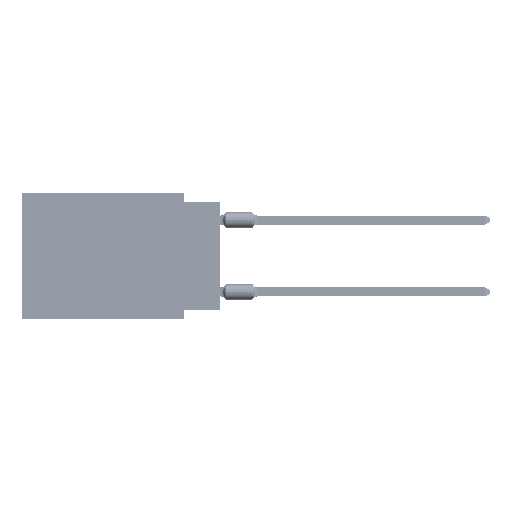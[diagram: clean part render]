
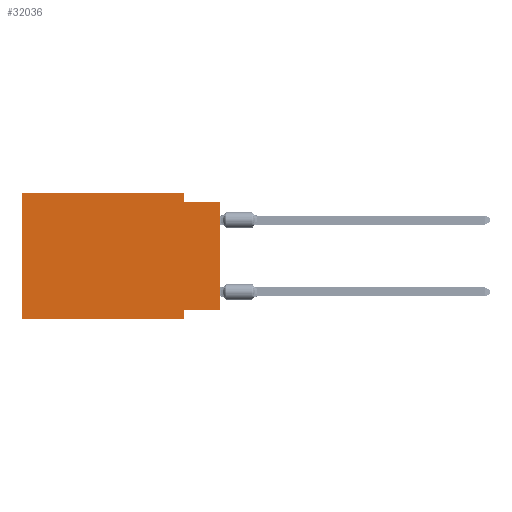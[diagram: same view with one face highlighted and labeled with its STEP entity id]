
A CAD part, left-side view. The second image highlights one B-rep face of the part: STEP entity #32036.
In plain terms, the highlighted planar face has unit normal (-1, 0, 0).
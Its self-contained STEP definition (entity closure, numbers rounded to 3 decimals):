
#431 = EDGE_CURVE ( 'NONE', #12247, #24004, #106293, .T. ) ;
#2744 = LINE ( 'NONE', #40920, #111306 ) ;
#5937 = DIRECTION ( 'NONE',  ( 0., -1., 0. ) ) ;
#11115 = CARTESIAN_POINT ( 'NONE',  ( 0., 0., -0.635 ) ) ;
#11215 = VERTEX_POINT ( 'NONE', #73390 ) ;
#11297 = VECTOR ( 'NONE', #75591, 1000. ) ;
#12247 = VERTEX_POINT ( 'NONE', #87187 ) ;
#15768 = CARTESIAN_POINT ( 'NONE',  ( 0., 13.97, 0. ) ) ;
#18069 = EDGE_CURVE ( 'NONE', #34538, #65398, #113765, .T. ) ;
#20602 = FACE_OUTER_BOUND ( 'NONE', #29272, .T. ) ;
#21909 = DIRECTION ( 'NONE',  ( 0., 0., 1. ) ) ;
#23655 = DIRECTION ( 'NONE',  ( 0., 0., -1. ) ) ;
#24004 = VERTEX_POINT ( 'NONE', #77155 ) ;
#27257 = ORIENTED_EDGE ( 'NONE', *, *, #98358, .F. ) ;
#28220 = LINE ( 'NONE', #68195, #44627 ) ;
#29272 = EDGE_LOOP ( 'NONE', ( #40018, #65477, #35209, #44432, #27257, #119231, #104005, #34527 ) ) ;
#30607 = CARTESIAN_POINT ( 'NONE',  ( 0., 13.97, 0. ) ) ;
#32036 = ADVANCED_FACE ( 'NONE', ( #20602 ), #96289, .F. ) ;
#32522 = CARTESIAN_POINT ( 'NONE',  ( 0., 0., -8.255 ) ) ;
#32680 = CARTESIAN_POINT ( 'NONE',  ( 0., 2.54, 0. ) ) ;
#34527 = ORIENTED_EDGE ( 'NONE', *, *, #18069, .F. ) ;
#34538 = VERTEX_POINT ( 'NONE', #32522 ) ;
#35209 = ORIENTED_EDGE ( 'NONE', *, *, #67756, .F. ) ;
#35765 = VECTOR ( 'NONE', #70231, 1000. ) ;
#39027 = VECTOR ( 'NONE', #5937, 1000. ) ;
#39082 = DIRECTION ( 'NONE',  ( 0., 0., -1. ) ) ;
#40018 = ORIENTED_EDGE ( 'NONE', *, *, #86306, .T. ) ;
#40446 = DIRECTION ( 'NONE',  ( 0., -1., 0. ) ) ;
#40472 = VERTEX_POINT ( 'NONE', #11115 ) ;
#40532 = CARTESIAN_POINT ( 'NONE',  ( 0., 2.54, -0.635 ) ) ;
#40920 = CARTESIAN_POINT ( 'NONE',  ( 0., 2.54, -8.89 ) ) ;
#43041 = VERTEX_POINT ( 'NONE', #73592 ) ;
#44149 = CARTESIAN_POINT ( 'NONE',  ( 0., 2.54, -8.255 ) ) ;
#44432 = ORIENTED_EDGE ( 'NONE', *, *, #431, .F. ) ;
#44627 = VECTOR ( 'NONE', #105753, 1000. ) ;
#47868 = VECTOR ( 'NONE', #40446, 1000. ) ;
#49040 = CARTESIAN_POINT ( 'NONE',  ( 0., 0., 0. ) ) ;
#50225 = LINE ( 'NONE', #49040, #109811 ) ;
#51982 = VERTEX_POINT ( 'NONE', #40532 ) ;
#54453 = AXIS2_PLACEMENT_3D ( 'NONE', #77192, #76007, #39082 ) ;
#60740 = EDGE_CURVE ( 'NONE', #65398, #43041, #2744, .T. ) ;
#61965 = LINE ( 'NONE', #99494, #39027 ) ;
#65398 = VERTEX_POINT ( 'NONE', #44149 ) ;
#65477 = ORIENTED_EDGE ( 'NONE', *, *, #99718, .F. ) ;
#67756 = EDGE_CURVE ( 'NONE', #24004, #51982, #88086, .T. ) ;
#68195 = CARTESIAN_POINT ( 'NONE',  ( 0., 13.97, -8.89 ) ) ;
#70231 = DIRECTION ( 'NONE',  ( 0., 0., -1. ) ) ;
#70576 = DIRECTION ( 'NONE',  ( 0., 0., 1. ) ) ;
#73390 = CARTESIAN_POINT ( 'NONE',  ( 0., 13.97, -8.89 ) ) ;
#73592 = CARTESIAN_POINT ( 'NONE',  ( 0., 2.54, -8.89 ) ) ;
#75591 = DIRECTION ( 'NONE',  ( 0., 1., 0. ) ) ;
#76007 = DIRECTION ( 'NONE',  ( 1., 0., 0. ) ) ;
#77155 = CARTESIAN_POINT ( 'NONE',  ( 0., 2.54, 0. ) ) ;
#77192 = CARTESIAN_POINT ( 'NONE',  ( 0., 13.97, 0. ) ) ;
#82605 = EDGE_CURVE ( 'NONE', #11215, #43041, #28220, .T. ) ;
#86306 = EDGE_CURVE ( 'NONE', #34538, #40472, #50225, .T. ) ;
#87187 = CARTESIAN_POINT ( 'NONE',  ( 0., 13.97, 0. ) ) ;
#88086 = LINE ( 'NONE', #32680, #35765 ) ;
#96289 = PLANE ( 'NONE',  #54453 ) ;
#98358 = EDGE_CURVE ( 'NONE', #11215, #12247, #100084, .T. ) ;
#99494 = CARTESIAN_POINT ( 'NONE',  ( 0., 0., -0.635 ) ) ;
#99718 = EDGE_CURVE ( 'NONE', #51982, #40472, #61965, .T. ) ;
#100084 = LINE ( 'NONE', #15768, #121466 ) ;
#103302 = CARTESIAN_POINT ( 'NONE',  ( 0., 0., -8.255 ) ) ;
#104005 = ORIENTED_EDGE ( 'NONE', *, *, #60740, .F. ) ;
#105753 = DIRECTION ( 'NONE',  ( 0., -1., 0. ) ) ;
#106293 = LINE ( 'NONE', #30607, #47868 ) ;
#109811 = VECTOR ( 'NONE', #21909, 1000. ) ;
#111306 = VECTOR ( 'NONE', #23655, 1000. ) ;
#113765 = LINE ( 'NONE', #103302, #11297 ) ;
#119231 = ORIENTED_EDGE ( 'NONE', *, *, #82605, .T. ) ;
#121466 = VECTOR ( 'NONE', #70576, 1000. ) ;
